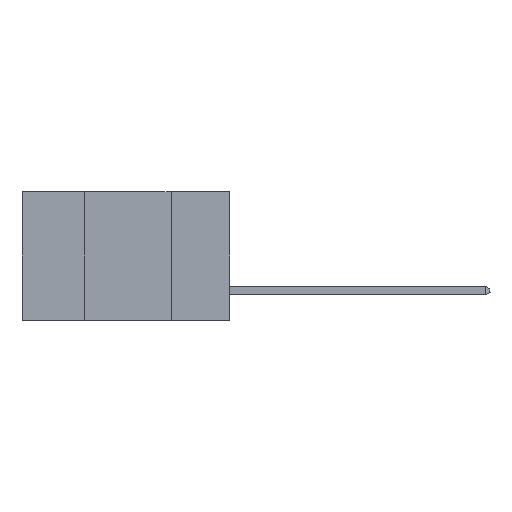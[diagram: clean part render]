
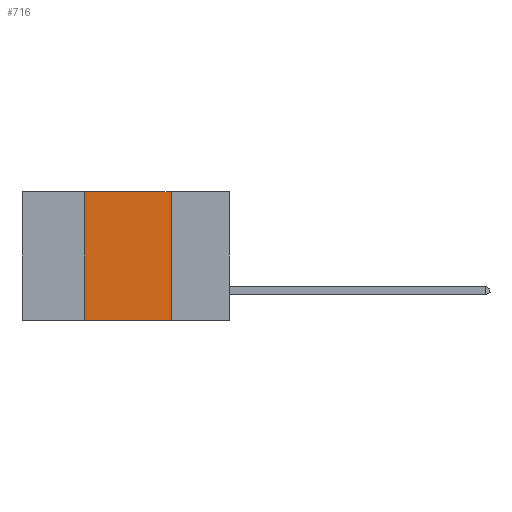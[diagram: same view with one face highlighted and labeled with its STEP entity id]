
A CAD part, left-side view. The second image highlights one B-rep face of the part: STEP entity #716.
In plain terms, the highlighted planar face has unit normal (-1, 0, 0).
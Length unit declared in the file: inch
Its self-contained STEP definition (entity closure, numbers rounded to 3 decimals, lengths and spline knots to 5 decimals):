
#406 = ORIENTED_EDGE ( 'NONE', *, *, #6272, .F. ) ;
#716 = ADVANCED_FACE ( 'NONE', ( #8179 ), #4920, .F. ) ;
#1190 = EDGE_CURVE ( 'NONE', #5099, #7106, #10342, .T. ) ;
#1667 = CARTESIAN_POINT ( 'NONE',  ( 0., 0.6, -0.37 ) ) ;
#1915 = CARTESIAN_POINT ( 'NONE',  ( 0., 0.6, 0. ) ) ;
#2243 = VECTOR ( 'NONE', #9264, 39.37008 ) ;
#2398 = DIRECTION ( 'NONE',  ( 0., 0., -1. ) ) ;
#2417 = DIRECTION ( 'NONE',  ( 0., 0., 1. ) ) ;
#3969 = LINE ( 'NONE', #10510, #5228 ) ;
#3975 = CARTESIAN_POINT ( 'NONE',  ( 0., 0.42, 0. ) ) ;
#4614 = CARTESIAN_POINT ( 'NONE',  ( 0., 0.17, 0. ) ) ;
#4627 = VECTOR ( 'NONE', #4981, 39.37008 ) ;
#4920 = PLANE ( 'NONE',  #9076 ) ;
#4964 = EDGE_CURVE ( 'NONE', #9920, #7106, #9885, .T. ) ;
#4981 = DIRECTION ( 'NONE',  ( 0., -1., 0. ) ) ;
#5089 = DIRECTION ( 'NONE',  ( 0., -1., 0. ) ) ;
#5099 = VERTEX_POINT ( 'NONE', #5689 ) ;
#5228 = VECTOR ( 'NONE', #2417, 39.37008 ) ;
#5346 = ORIENTED_EDGE ( 'NONE', *, *, #8555, .F. ) ;
#5689 = CARTESIAN_POINT ( 'NONE',  ( 0., 0.42, -0.37 ) ) ;
#6272 = EDGE_CURVE ( 'NONE', #5099, #9457, #3969, .T. ) ;
#6407 = DIRECTION ( 'NONE',  ( 1., 0., 0. ) ) ;
#6481 = CARTESIAN_POINT ( 'NONE',  ( 0., 0.6, 0. ) ) ;
#7106 = VERTEX_POINT ( 'NONE', #8896 ) ;
#7309 = LINE ( 'NONE', #1915, #8345 ) ;
#8179 = FACE_OUTER_BOUND ( 'NONE', #8767, .T. ) ;
#8197 = ORIENTED_EDGE ( 'NONE', *, *, #1190, .T. ) ;
#8345 = VECTOR ( 'NONE', #5089, 39.37008 ) ;
#8555 = EDGE_CURVE ( 'NONE', #9457, #9920, #7309, .T. ) ;
#8767 = EDGE_LOOP ( 'NONE', ( #10498, #5346, #406, #8197 ) ) ;
#8896 = CARTESIAN_POINT ( 'NONE',  ( 0., 0.17, -0.37 ) ) ;
#9076 = AXIS2_PLACEMENT_3D ( 'NONE', #6481, #6407, #2398 ) ;
#9264 = DIRECTION ( 'NONE',  ( 0., 0., -1. ) ) ;
#9409 = CARTESIAN_POINT ( 'NONE',  ( 0., 0.17, 0. ) ) ;
#9457 = VERTEX_POINT ( 'NONE', #3975 ) ;
#9885 = LINE ( 'NONE', #9409, #2243 ) ;
#9920 = VERTEX_POINT ( 'NONE', #4614 ) ;
#10342 = LINE ( 'NONE', #1667, #4627 ) ;
#10498 = ORIENTED_EDGE ( 'NONE', *, *, #4964, .F. ) ;
#10510 = CARTESIAN_POINT ( 'NONE',  ( 0., 0.42, 0. ) ) ;
